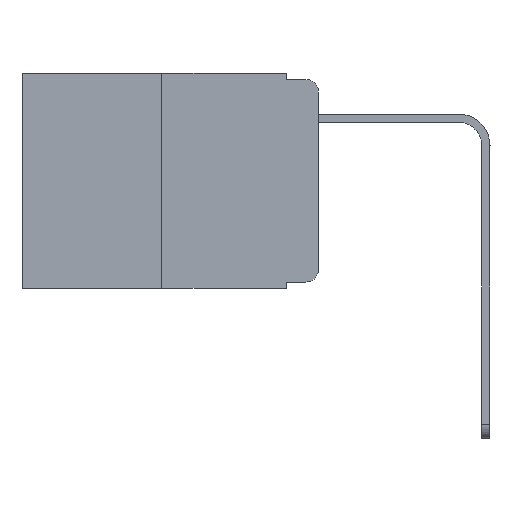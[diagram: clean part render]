
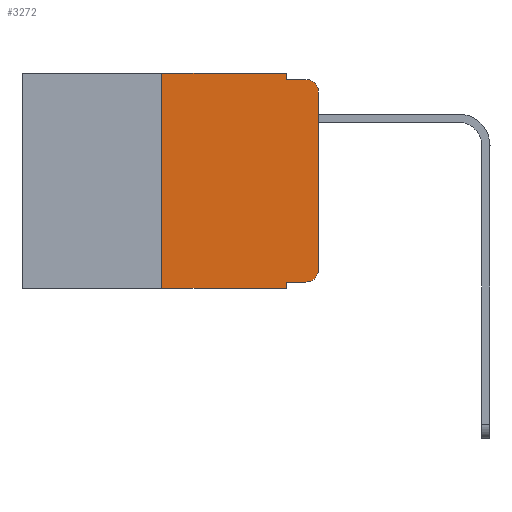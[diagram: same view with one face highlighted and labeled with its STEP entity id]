
A CAD part, left-side view. The second image highlights one B-rep face of the part: STEP entity #3272.
In plain terms, the highlighted planar face has unit normal (-1, 0, 0).
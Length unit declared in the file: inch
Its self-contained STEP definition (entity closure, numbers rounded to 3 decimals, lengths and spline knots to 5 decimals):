
#92 = VECTOR ( 'NONE', #12681, 39.37008 ) ;
#249 = CARTESIAN_POINT ( 'NONE',  ( 0., 0.473, 0. ) ) ;
#299 = DIRECTION ( 'NONE',  ( 0., 0., -1. ) ) ;
#583 = CARTESIAN_POINT ( 'NONE',  ( 0., 0.051, -0.343 ) ) ;
#690 = EDGE_CURVE ( 'NONE', #5690, #4147, #1074, .T. ) ;
#1074 = LINE ( 'NONE', #1673, #4834 ) ;
#1187 = LINE ( 'NONE', #14055, #11172 ) ;
#1229 = LINE ( 'NONE', #1815, #92 ) ;
#1314 = DIRECTION ( 'NONE',  ( 1., 0., 0. ) ) ;
#1410 = CARTESIAN_POINT ( 'NONE',  ( 0., 0.25, 0. ) ) ;
#1471 = PLANE ( 'NONE',  #14199 ) ;
#1673 = CARTESIAN_POINT ( 'NONE',  ( 0., 0.051, 0. ) ) ;
#1815 = CARTESIAN_POINT ( 'NONE',  ( 0., 0.051, 0. ) ) ;
#1838 = EDGE_CURVE ( 'NONE', #6923, #5690, #13833, .T. ) ;
#1946 = VERTEX_POINT ( 'NONE', #6483 ) ;
#2039 = EDGE_CURVE ( 'NONE', #7222, #6923, #6141, .T. ) ;
#2277 = VERTEX_POINT ( 'NONE', #3367 ) ;
#2944 = VECTOR ( 'NONE', #10118, 39.37008 ) ;
#2946 = EDGE_CURVE ( 'NONE', #7249, #11269, #1187, .T. ) ;
#3007 = LINE ( 'NONE', #6365, #7542 ) ;
#3022 = ORIENTED_EDGE ( 'NONE', *, *, #2039, .F. ) ;
#3272 = ADVANCED_FACE ( 'NONE', ( #5137 ), #1471, .F. ) ;
#3367 = CARTESIAN_POINT ( 'NONE',  ( 0., 0., -0.313 ) ) ;
#3652 = CIRCLE ( 'NONE', #12029, 0.02 ) ;
#3710 = VECTOR ( 'NONE', #10261, 39.37008 ) ;
#3740 = LINE ( 'NONE', #12146, #9940 ) ;
#4144 = ORIENTED_EDGE ( 'NONE', *, *, #10849, .T. ) ;
#4147 = VERTEX_POINT ( 'NONE', #6897 ) ;
#4447 = CARTESIAN_POINT ( 'NONE',  ( 0., 0.02, -0.03 ) ) ;
#4834 = VECTOR ( 'NONE', #11632, 39.37008 ) ;
#4894 = DIRECTION ( 'NONE',  ( 0., -1., 0. ) ) ;
#5137 = FACE_OUTER_BOUND ( 'NONE', #12705, .T. ) ;
#5352 = ORIENTED_EDGE ( 'NONE', *, *, #2946, .T. ) ;
#5490 = EDGE_CURVE ( 'NONE', #11269, #2277, #14455, .T. ) ;
#5506 = CARTESIAN_POINT ( 'NONE',  ( 0., 0.25, -0.343 ) ) ;
#5528 = ORIENTED_EDGE ( 'NONE', *, *, #7276, .T. ) ;
#5659 = DIRECTION ( 'NONE',  ( -1., 0., 0. ) ) ;
#5690 = VERTEX_POINT ( 'NONE', #14613 ) ;
#5888 = AXIS2_PLACEMENT_3D ( 'NONE', #11737, #7006, #10673 ) ;
#6141 = LINE ( 'NONE', #11191, #2944 ) ;
#6221 = EDGE_CURVE ( 'NONE', #4147, #1946, #3740, .T. ) ;
#6365 = CARTESIAN_POINT ( 'NONE',  ( 0., 0.473, -0.343 ) ) ;
#6483 = CARTESIAN_POINT ( 'NONE',  ( 0., 0.02, -0.01 ) ) ;
#6897 = CARTESIAN_POINT ( 'NONE',  ( 0., 0.051, -0.01 ) ) ;
#6923 = VERTEX_POINT ( 'NONE', #1410 ) ;
#7006 = DIRECTION ( 'NONE',  ( -1., 0., 0. ) ) ;
#7222 = VERTEX_POINT ( 'NONE', #5506 ) ;
#7249 = VERTEX_POINT ( 'NONE', #11490 ) ;
#7276 = EDGE_CURVE ( 'NONE', #2277, #9213, #10086, .T. ) ;
#7542 = VECTOR ( 'NONE', #12402, 39.37008 ) ;
#8140 = DIRECTION ( 'NONE',  ( 0., -1., 0. ) ) ;
#8806 = ORIENTED_EDGE ( 'NONE', *, *, #690, .F. ) ;
#8999 = VERTEX_POINT ( 'NONE', #583 ) ;
#9110 = ORIENTED_EDGE ( 'NONE', *, *, #13308, .F. ) ;
#9213 = VERTEX_POINT ( 'NONE', #11705 ) ;
#9528 = CARTESIAN_POINT ( 'NONE',  ( 0., 0.02, -0.333 ) ) ;
#9940 = VECTOR ( 'NONE', #4894, 39.37008 ) ;
#10086 = LINE ( 'NONE', #15030, #3710 ) ;
#10118 = DIRECTION ( 'NONE',  ( 0., 0., 1. ) ) ;
#10261 = DIRECTION ( 'NONE',  ( 0., 0., 1. ) ) ;
#10280 = ORIENTED_EDGE ( 'NONE', *, *, #1838, .F. ) ;
#10673 = DIRECTION ( 'NONE',  ( 0., 0., -1. ) ) ;
#10716 = DIRECTION ( 'NONE',  ( 0., -1., 0. ) ) ;
#10849 = EDGE_CURVE ( 'NONE', #7222, #8999, #3007, .T. ) ;
#11172 = VECTOR ( 'NONE', #8140, 39.37008 ) ;
#11191 = CARTESIAN_POINT ( 'NONE',  ( 0., 0.25, 0. ) ) ;
#11234 = VECTOR ( 'NONE', #10716, 39.37008 ) ;
#11269 = VERTEX_POINT ( 'NONE', #9528 ) ;
#11490 = CARTESIAN_POINT ( 'NONE',  ( 0., 0.051, -0.333 ) ) ;
#11632 = DIRECTION ( 'NONE',  ( 0., 0., -1. ) ) ;
#11705 = CARTESIAN_POINT ( 'NONE',  ( 0., 0., -0.03 ) ) ;
#11737 = CARTESIAN_POINT ( 'NONE',  ( 0., 0.02, -0.313 ) ) ;
#12029 = AXIS2_PLACEMENT_3D ( 'NONE', #4447, #5659, #12226 ) ;
#12146 = CARTESIAN_POINT ( 'NONE',  ( 0., 0.051, -0.01 ) ) ;
#12226 = DIRECTION ( 'NONE',  ( 0., 0., -1. ) ) ;
#12402 = DIRECTION ( 'NONE',  ( 0., -1., 0. ) ) ;
#12656 = ORIENTED_EDGE ( 'NONE', *, *, #14008, .T. ) ;
#12681 = DIRECTION ( 'NONE',  ( 0., 0., -1. ) ) ;
#12705 = EDGE_LOOP ( 'NONE', ( #5528, #12656, #14559, #8806, #10280, #3022, #4144, #9110, #5352, #15276 ) ) ;
#13308 = EDGE_CURVE ( 'NONE', #7249, #8999, #1229, .T. ) ;
#13833 = LINE ( 'NONE', #14228, #11234 ) ;
#14008 = EDGE_CURVE ( 'NONE', #9213, #1946, #3652, .T. ) ;
#14055 = CARTESIAN_POINT ( 'NONE',  ( 0., 0.051, -0.333 ) ) ;
#14199 = AXIS2_PLACEMENT_3D ( 'NONE', #249, #1314, #299 ) ;
#14228 = CARTESIAN_POINT ( 'NONE',  ( 0., 0.473, 0. ) ) ;
#14455 = CIRCLE ( 'NONE', #5888, 0.02 ) ;
#14559 = ORIENTED_EDGE ( 'NONE', *, *, #6221, .F. ) ;
#14613 = CARTESIAN_POINT ( 'NONE',  ( 0., 0.051, 0. ) ) ;
#15030 = CARTESIAN_POINT ( 'NONE',  ( 0., 0., 0. ) ) ;
#15276 = ORIENTED_EDGE ( 'NONE', *, *, #5490, .T. ) ;
